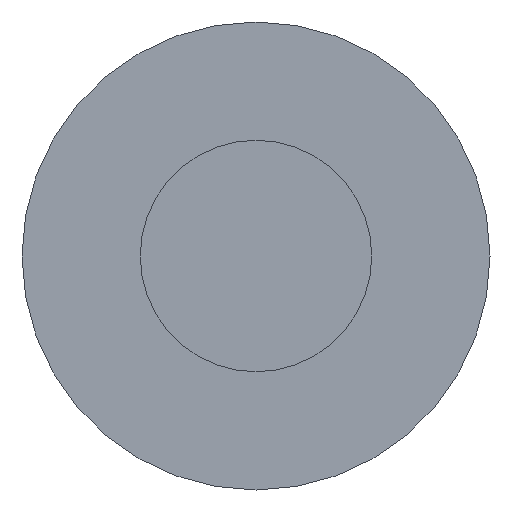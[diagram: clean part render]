
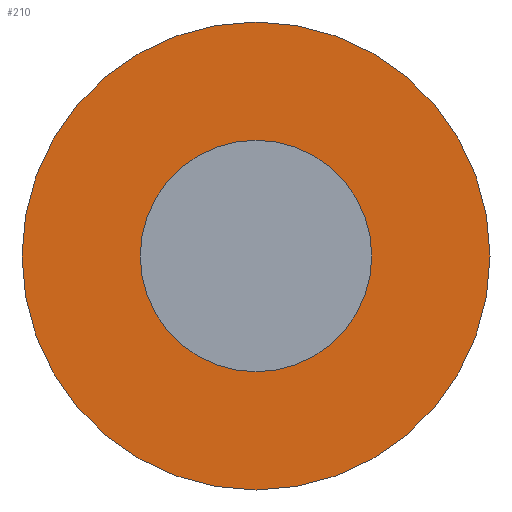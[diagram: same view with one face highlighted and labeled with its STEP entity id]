
A CAD part, front view. The second image highlights one B-rep face of the part: STEP entity #210.
In plain terms, the highlighted planar face has unit normal (0, -1, 0).
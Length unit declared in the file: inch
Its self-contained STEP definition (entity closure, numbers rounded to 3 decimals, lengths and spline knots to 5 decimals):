
#3 = DIRECTION ( 'NONE',  ( 0., -1., 0. ) ) ;
#5 = EDGE_LOOP ( 'NONE', ( #136, #193 ) ) ;
#10 = VERTEX_POINT ( 'NONE', #86 ) ;
#30 = CARTESIAN_POINT ( 'NONE',  ( 0., 1., -0.40437 ) ) ;
#31 = DIRECTION ( 'NONE',  ( 0., 0., -1. ) ) ;
#36 = CARTESIAN_POINT ( 'NONE',  ( 0., 1., 0. ) ) ;
#38 = CARTESIAN_POINT ( 'NONE',  ( 0., 1., 0. ) ) ;
#39 = DIRECTION ( 'NONE',  ( 0., 0., -1. ) ) ;
#44 = DIRECTION ( 'NONE',  ( 0., 0., -1. ) ) ;
#45 = VERTEX_POINT ( 'NONE', #84 ) ;
#47 = CARTESIAN_POINT ( 'NONE',  ( 0., 1., 0. ) ) ;
#53 = EDGE_CURVE ( 'NONE', #45, #10, #87, .T. ) ;
#67 = EDGE_CURVE ( 'NONE', #139, #255, #97, .T. ) ;
#74 = AXIS2_PLACEMENT_3D ( 'NONE', #36, #231, #104 ) ;
#84 = CARTESIAN_POINT ( 'NONE',  ( 0., 1., 0.2 ) ) ;
#86 = CARTESIAN_POINT ( 'NONE',  ( 0., 1., -0.2 ) ) ;
#87 = CIRCLE ( 'NONE', #280, 0.2 ) ;
#90 = AXIS2_PLACEMENT_3D ( 'NONE', #208, #99, #229 ) ;
#95 = EDGE_CURVE ( 'NONE', #255, #139, #174, .T. ) ;
#97 = CIRCLE ( 'NONE', #74, 0.40437 ) ;
#99 = DIRECTION ( 'NONE',  ( 0., -1., 0. ) ) ;
#104 = DIRECTION ( 'NONE',  ( 0., 0., -1. ) ) ;
#136 = ORIENTED_EDGE ( 'NONE', *, *, #194, .F. ) ;
#139 = VERTEX_POINT ( 'NONE', #260 ) ;
#142 = FACE_OUTER_BOUND ( 'NONE', #227, .T. ) ;
#159 = CIRCLE ( 'NONE', #90, 0.2 ) ;
#172 = ORIENTED_EDGE ( 'NONE', *, *, #95, .T. ) ;
#174 = CIRCLE ( 'NONE', #176, 0.40437 ) ;
#176 = AXIS2_PLACEMENT_3D ( 'NONE', #221, #257, #44 ) ;
#181 = PLANE ( 'NONE',  #217 ) ;
#188 = ORIENTED_EDGE ( 'NONE', *, *, #67, .T. ) ;
#193 = ORIENTED_EDGE ( 'NONE', *, *, #53, .F. ) ;
#194 = EDGE_CURVE ( 'NONE', #10, #45, #159, .T. ) ;
#205 = FACE_BOUND ( 'NONE', #5, .T. ) ;
#208 = CARTESIAN_POINT ( 'NONE',  ( 0., 1., 0. ) ) ;
#210 = ADVANCED_FACE ( 'NONE', ( #142, #205 ), #181, .T. ) ;
#217 = AXIS2_PLACEMENT_3D ( 'NONE', #47, #3, #31 ) ;
#221 = CARTESIAN_POINT ( 'NONE',  ( 0., 1., 0. ) ) ;
#227 = EDGE_LOOP ( 'NONE', ( #172, #188 ) ) ;
#229 = DIRECTION ( 'NONE',  ( 0., 0., -1. ) ) ;
#231 = DIRECTION ( 'NONE',  ( 0., -1., 0. ) ) ;
#234 = DIRECTION ( 'NONE',  ( 0., -1., 0. ) ) ;
#255 = VERTEX_POINT ( 'NONE', #30 ) ;
#257 = DIRECTION ( 'NONE',  ( 0., -1., 0. ) ) ;
#260 = CARTESIAN_POINT ( 'NONE',  ( 0., 1., 0.40437 ) ) ;
#280 = AXIS2_PLACEMENT_3D ( 'NONE', #38, #234, #39 ) ;
